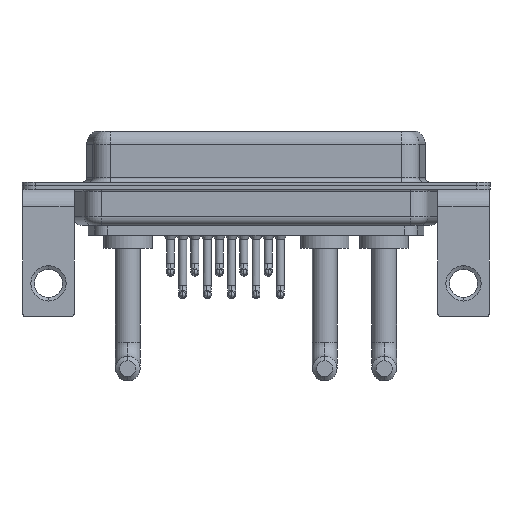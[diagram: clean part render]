
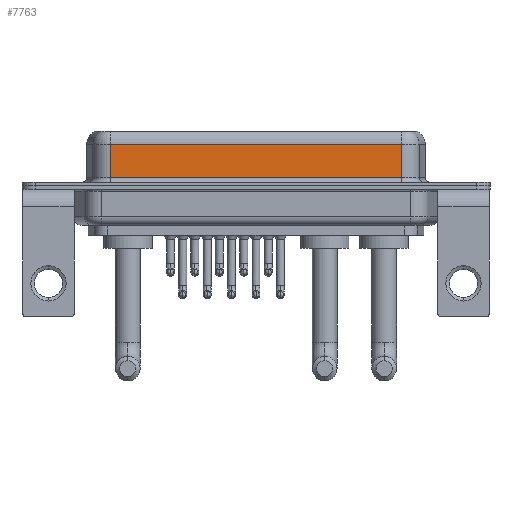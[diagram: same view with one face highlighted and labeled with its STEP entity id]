
A CAD part, front view. The second image highlights one B-rep face of the part: STEP entity #7763.
In plain terms, the highlighted planar face has unit normal (0, -1, 0).
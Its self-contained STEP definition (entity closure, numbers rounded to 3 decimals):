
#959 = PLANE ( 'NONE',  #10392 ) ;
#1581 = CARTESIAN_POINT ( 'NONE',  ( 40.037, -3.95, 4.65 ) ) ;
#2209 = ORIENTED_EDGE ( 'NONE', *, *, #17907, .T. ) ;
#2465 = VECTOR ( 'NONE', #12621, 1000. ) ;
#2480 = VECTOR ( 'NONE', #3275, 1000. ) ;
#2911 = ORIENTED_EDGE ( 'NONE', *, *, #13155, .F. ) ;
#3275 = DIRECTION ( 'NONE',  ( -1., 0., 0. ) ) ;
#3564 = CARTESIAN_POINT ( 'NONE',  ( 40.037, -3.95, 6.4 ) ) ;
#4469 = VECTOR ( 'NONE', #15738, 1000. ) ;
#4693 = LINE ( 'NONE', #13942, #14033 ) ;
#4973 = LINE ( 'NONE', #3564, #2465 ) ;
#5266 = ORIENTED_EDGE ( 'NONE', *, *, #17939, .T. ) ;
#5921 = FACE_OUTER_BOUND ( 'NONE', #17697, .T. ) ;
#7538 = DIRECTION ( 'NONE',  ( 0., 1., 0. ) ) ;
#7763 = ADVANCED_FACE ( 'NONE', ( #5921 ), #959, .F. ) ;
#7879 = VERTEX_POINT ( 'NONE', #11352 ) ;
#9208 = CARTESIAN_POINT ( 'NONE',  ( 7.013, -3.95, 6.4 ) ) ;
#9254 = CARTESIAN_POINT ( 'NONE',  ( 40.037, -3.95, 4.65 ) ) ;
#9348 = CARTESIAN_POINT ( 'NONE',  ( 40.037, -3.95, 6.4 ) ) ;
#9632 = LINE ( 'NONE', #1581, #2480 ) ;
#10392 = AXIS2_PLACEMENT_3D ( 'NONE', #9348, #7538, #15479 ) ;
#11352 = CARTESIAN_POINT ( 'NONE',  ( 7.013, -3.95, 0.9 ) ) ;
#12621 = DIRECTION ( 'NONE',  ( 0., 0., -1. ) ) ;
#13155 = EDGE_CURVE ( 'NONE', #17418, #15289, #4973, .T. ) ;
#13831 = LINE ( 'NONE', #9208, #4469 ) ;
#13942 = CARTESIAN_POINT ( 'NONE',  ( 40.037, -3.95, 0.9 ) ) ;
#14033 = VECTOR ( 'NONE', #15654, 1000. ) ;
#15289 = VERTEX_POINT ( 'NONE', #18505 ) ;
#15316 = CARTESIAN_POINT ( 'NONE',  ( 7.013, -3.95, 4.65 ) ) ;
#15479 = DIRECTION ( 'NONE',  ( 0., 0., 1. ) ) ;
#15654 = DIRECTION ( 'NONE',  ( 1., 0., 0. ) ) ;
#15738 = DIRECTION ( 'NONE',  ( 0., 0., -1. ) ) ;
#16807 = VERTEX_POINT ( 'NONE', #15316 ) ;
#17418 = VERTEX_POINT ( 'NONE', #9254 ) ;
#17697 = EDGE_LOOP ( 'NONE', ( #2911, #5266, #19579, #2209 ) ) ;
#17907 = EDGE_CURVE ( 'NONE', #7879, #15289, #4693, .T. ) ;
#17939 = EDGE_CURVE ( 'NONE', #17418, #16807, #9632, .T. ) ;
#18505 = CARTESIAN_POINT ( 'NONE',  ( 40.037, -3.95, 0.9 ) ) ;
#19579 = ORIENTED_EDGE ( 'NONE', *, *, #19638, .T. ) ;
#19638 = EDGE_CURVE ( 'NONE', #16807, #7879, #13831, .T. ) ;
